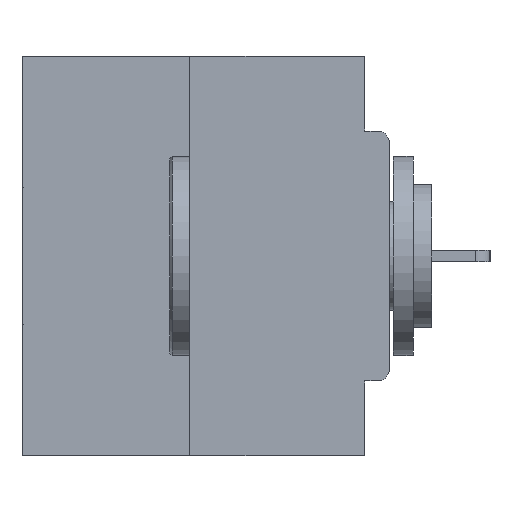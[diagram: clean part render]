
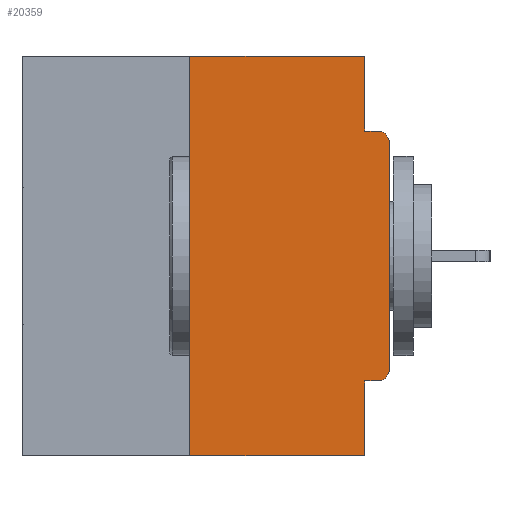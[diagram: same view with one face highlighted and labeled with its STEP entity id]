
A CAD part, left-side view. The second image highlights one B-rep face of the part: STEP entity #20359.
In plain terms, the highlighted planar face has unit normal (-1, 0, 0).
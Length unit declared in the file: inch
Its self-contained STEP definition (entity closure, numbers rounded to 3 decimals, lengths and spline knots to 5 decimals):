
#432 = CARTESIAN_POINT ( 'NONE',  ( 0., 0.46, 0. ) ) ;
#1217 = VERTEX_POINT ( 'NONE', #30481 ) ;
#1890 = ORIENTED_EDGE ( 'NONE', *, *, #9184, .F. ) ;
#2022 = VECTOR ( 'NONE', #11544, 39.37008 ) ;
#2944 = CARTESIAN_POINT ( 'NONE',  ( 0., 0.031, 0. ) ) ;
#3362 = EDGE_CURVE ( 'NONE', #23282, #27068, #24286, .T. ) ;
#3387 = CARTESIAN_POINT ( 'NONE',  ( 0., 0.25, 0. ) ) ;
#3507 = DIRECTION ( 'NONE',  ( 1., 0., 0. ) ) ;
#3665 = CARTESIAN_POINT ( 'NONE',  ( 0., 0.015, -0.0935 ) ) ;
#4256 = ORIENTED_EDGE ( 'NONE', *, *, #26678, .F. ) ;
#4386 = CARTESIAN_POINT ( 'NONE',  ( 0., 0.031, -0.0935 ) ) ;
#4632 = EDGE_CURVE ( 'NONE', #31256, #17611, #22235, .T. ) ;
#4964 = ORIENTED_EDGE ( 'NONE', *, *, #4632, .T. ) ;
#6059 = ORIENTED_EDGE ( 'NONE', *, *, #3362, .F. ) ;
#6863 = CARTESIAN_POINT ( 'NONE',  ( 0., 0.25, -0.5 ) ) ;
#6977 = DIRECTION ( 'NONE',  ( 0., -1., 0. ) ) ;
#7019 = CIRCLE ( 'NONE', #14661, 0.015 ) ;
#7305 = LINE ( 'NONE', #12456, #20543 ) ;
#8032 = EDGE_LOOP ( 'NONE', ( #20685, #8224, #32258, #1890, #4256, #25086, #4964, #18625, #28599, #6059 ) ) ;
#8224 = ORIENTED_EDGE ( 'NONE', *, *, #12837, .F. ) ;
#9184 = EDGE_CURVE ( 'NONE', #21412, #1217, #30775, .T. ) ;
#9784 = CARTESIAN_POINT ( 'NONE',  ( 0., 0.031, -0.5 ) ) ;
#10576 = VECTOR ( 'NONE', #12687, 39.37008 ) ;
#10680 = DIRECTION ( 'NONE',  ( 0., 0., -1. ) ) ;
#10930 = CARTESIAN_POINT ( 'NONE',  ( 0., 0.031, 0. ) ) ;
#11003 = FACE_OUTER_BOUND ( 'NONE', #8032, .T. ) ;
#11296 = CIRCLE ( 'NONE', #20558, 0.015 ) ;
#11544 = DIRECTION ( 'NONE',  ( 0., -1., 0. ) ) ;
#11595 = EDGE_CURVE ( 'NONE', #25664, #23282, #16672, .T. ) ;
#12002 = VERTEX_POINT ( 'NONE', #3665 ) ;
#12109 = EDGE_CURVE ( 'NONE', #17611, #12002, #11296, .T. ) ;
#12259 = CARTESIAN_POINT ( 'NONE',  ( 0., 0.031, -0.4065 ) ) ;
#12456 = CARTESIAN_POINT ( 'NONE',  ( 0., 0., -0.0935 ) ) ;
#12687 = DIRECTION ( 'NONE',  ( 0., 0., -1. ) ) ;
#12837 = EDGE_CURVE ( 'NONE', #19399, #25664, #26776, .T. ) ;
#13423 = CARTESIAN_POINT ( 'NONE',  ( 0., 0., -0.3915 ) ) ;
#13997 = DIRECTION ( 'NONE',  ( 0., 0., 1. ) ) ;
#14278 = DIRECTION ( 'NONE',  ( -1., 0., 0. ) ) ;
#14327 = EDGE_CURVE ( 'NONE', #19399, #1217, #21597, .T. ) ;
#14661 = AXIS2_PLACEMENT_3D ( 'NONE', #24169, #14278, #27246 ) ;
#14828 = LINE ( 'NONE', #33606, #25998 ) ;
#14992 = DIRECTION ( 'NONE',  ( 0., 1., 0. ) ) ;
#16672 = LINE ( 'NONE', #27081, #2022 ) ;
#17103 = VECTOR ( 'NONE', #29796, 39.37008 ) ;
#17355 = CARTESIAN_POINT ( 'NONE',  ( 0., 0.25, 0. ) ) ;
#17450 = CARTESIAN_POINT ( 'NONE',  ( 0., 0., 0. ) ) ;
#17611 = VERTEX_POINT ( 'NONE', #27288 ) ;
#18625 = ORIENTED_EDGE ( 'NONE', *, *, #12109, .T. ) ;
#19267 = VECTOR ( 'NONE', #13997, 39.37008 ) ;
#19399 = VERTEX_POINT ( 'NONE', #6863 ) ;
#19674 = DIRECTION ( 'NONE',  ( 0., 0., 1. ) ) ;
#20359 = ADVANCED_FACE ( 'NONE', ( #11003 ), #23839, .F. ) ;
#20543 = VECTOR ( 'NONE', #6977, 39.37008 ) ;
#20558 = AXIS2_PLACEMENT_3D ( 'NONE', #27544, #24987, #33348 ) ;
#20685 = ORIENTED_EDGE ( 'NONE', *, *, #11595, .F. ) ;
#21363 = DIRECTION ( 'NONE',  ( 0., 0., -1. ) ) ;
#21412 = VERTEX_POINT ( 'NONE', #12259 ) ;
#21418 = CARTESIAN_POINT ( 'NONE',  ( 0., 0.46, -0.5 ) ) ;
#21597 = LINE ( 'NONE', #21418, #17103 ) ;
#22051 = VECTOR ( 'NONE', #19674, 39.37008 ) ;
#22235 = LINE ( 'NONE', #17450, #22051 ) ;
#22555 = CARTESIAN_POINT ( 'NONE',  ( 0., 0.015, -0.4065 ) ) ;
#23282 = VERTEX_POINT ( 'NONE', #10930 ) ;
#23839 = PLANE ( 'NONE',  #24800 ) ;
#24169 = CARTESIAN_POINT ( 'NONE',  ( 0., 0.015, -0.3915 ) ) ;
#24259 = EDGE_CURVE ( 'NONE', #27285, #31256, #7019, .T. ) ;
#24286 = LINE ( 'NONE', #2944, #26929 ) ;
#24800 = AXIS2_PLACEMENT_3D ( 'NONE', #432, #3507, #10680 ) ;
#24987 = DIRECTION ( 'NONE',  ( -1., 0., 0. ) ) ;
#25086 = ORIENTED_EDGE ( 'NONE', *, *, #24259, .T. ) ;
#25664 = VERTEX_POINT ( 'NONE', #17355 ) ;
#25998 = VECTOR ( 'NONE', #14992, 39.37008 ) ;
#26650 = EDGE_CURVE ( 'NONE', #27068, #12002, #7305, .T. ) ;
#26678 = EDGE_CURVE ( 'NONE', #27285, #21412, #14828, .T. ) ;
#26776 = LINE ( 'NONE', #3387, #19267 ) ;
#26929 = VECTOR ( 'NONE', #21363, 39.37008 ) ;
#27068 = VERTEX_POINT ( 'NONE', #4386 ) ;
#27081 = CARTESIAN_POINT ( 'NONE',  ( 0., 0.46, 0. ) ) ;
#27246 = DIRECTION ( 'NONE',  ( 0., 0., -1. ) ) ;
#27285 = VERTEX_POINT ( 'NONE', #22555 ) ;
#27288 = CARTESIAN_POINT ( 'NONE',  ( 0., 0., -0.1085 ) ) ;
#27544 = CARTESIAN_POINT ( 'NONE',  ( 0., 0.015, -0.1085 ) ) ;
#28599 = ORIENTED_EDGE ( 'NONE', *, *, #26650, .F. ) ;
#29796 = DIRECTION ( 'NONE',  ( 0., -1., 0. ) ) ;
#30481 = CARTESIAN_POINT ( 'NONE',  ( 0., 0.031, -0.5 ) ) ;
#30775 = LINE ( 'NONE', #9784, #10576 ) ;
#31256 = VERTEX_POINT ( 'NONE', #13423 ) ;
#32258 = ORIENTED_EDGE ( 'NONE', *, *, #14327, .T. ) ;
#33348 = DIRECTION ( 'NONE',  ( 0., 0., -1. ) ) ;
#33606 = CARTESIAN_POINT ( 'NONE',  ( 0., 0., -0.4065 ) ) ;
